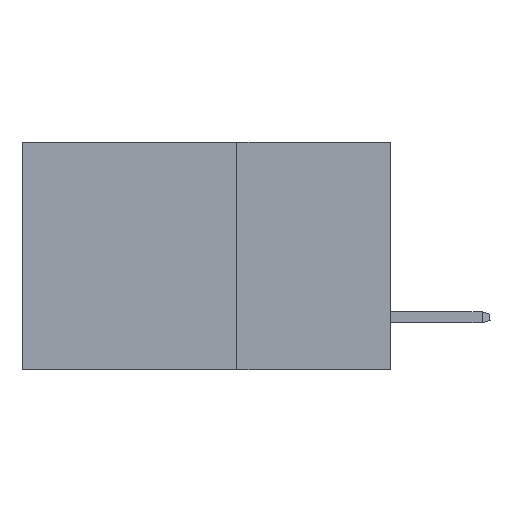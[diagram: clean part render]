
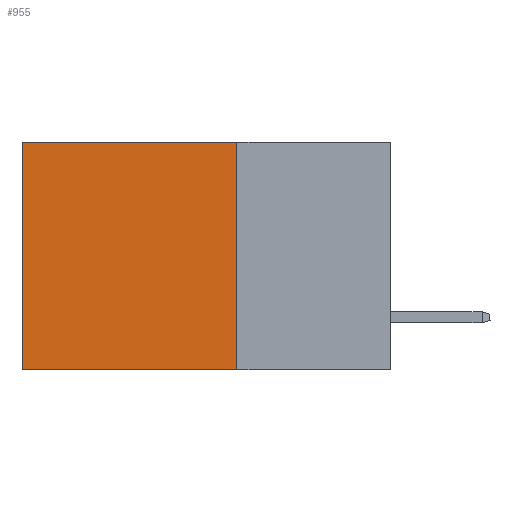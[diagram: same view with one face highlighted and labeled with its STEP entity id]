
A CAD part, left-side view. The second image highlights one B-rep face of the part: STEP entity #955.
In plain terms, the highlighted planar face has unit normal (-1, 0, 0).
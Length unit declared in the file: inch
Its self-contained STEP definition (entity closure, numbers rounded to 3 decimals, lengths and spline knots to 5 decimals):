
#955 = ADVANCED_FACE ( 'NONE', ( #3039 ), #11485, .F. ) ;
#1014 = EDGE_CURVE ( 'NONE', #9061, #15451, #6575, .T. ) ;
#3039 = FACE_OUTER_BOUND ( 'NONE', #24525, .T. ) ;
#3268 = VECTOR ( 'NONE', #10433, 39.37008 ) ;
#3573 = ORIENTED_EDGE ( 'NONE', *, *, #5496, .F. ) ;
#3801 = EDGE_CURVE ( 'NONE', #9061, #21072, #8751, .T. ) ;
#5016 = DIRECTION ( 'NONE',  ( 1., 0., 0. ) ) ;
#5496 = EDGE_CURVE ( 'NONE', #15451, #16793, #8081, .T. ) ;
#6575 = LINE ( 'NONE', #15434, #11398 ) ;
#7103 = VECTOR ( 'NONE', #8086, 39.37008 ) ;
#8081 = LINE ( 'NONE', #8127, #13527 ) ;
#8086 = DIRECTION ( 'NONE',  ( 0., 0., -1. ) ) ;
#8127 = CARTESIAN_POINT ( 'NONE',  ( 0.2875, 0.25, -0.37 ) ) ;
#8228 = ORIENTED_EDGE ( 'NONE', *, *, #3801, .T. ) ;
#8751 = LINE ( 'NONE', #21128, #3268 ) ;
#9061 = VERTEX_POINT ( 'NONE', #17352 ) ;
#10433 = DIRECTION ( 'NONE',  ( 0., 1., 0. ) ) ;
#10765 = ORIENTED_EDGE ( 'NONE', *, *, #24209, .T. ) ;
#11398 = VECTOR ( 'NONE', #17552, 39.37008 ) ;
#11485 = PLANE ( 'NONE',  #15212 ) ;
#13195 = CARTESIAN_POINT ( 'NONE',  ( 0.2875, 0.25, 0. ) ) ;
#13527 = VECTOR ( 'NONE', #26217, 39.37008 ) ;
#13822 = ORIENTED_EDGE ( 'NONE', *, *, #1014, .F. ) ;
#15212 = AXIS2_PLACEMENT_3D ( 'NONE', #13195, #5016, #25808 ) ;
#15434 = CARTESIAN_POINT ( 'NONE',  ( 0.2875, 0.25, 0. ) ) ;
#15451 = VERTEX_POINT ( 'NONE', #18130 ) ;
#16203 = CARTESIAN_POINT ( 'NONE',  ( 0.2875, 0.6, 0. ) ) ;
#16793 = VERTEX_POINT ( 'NONE', #17631 ) ;
#17352 = CARTESIAN_POINT ( 'NONE',  ( 0.2875, 0.25, 0. ) ) ;
#17552 = DIRECTION ( 'NONE',  ( 0., 0., -1. ) ) ;
#17631 = CARTESIAN_POINT ( 'NONE',  ( 0.2875, 0.6, -0.37 ) ) ;
#18130 = CARTESIAN_POINT ( 'NONE',  ( 0.2875, 0.25, -0.37 ) ) ;
#21072 = VERTEX_POINT ( 'NONE', #22028 ) ;
#21128 = CARTESIAN_POINT ( 'NONE',  ( 0.2875, 0.25, 0. ) ) ;
#22028 = CARTESIAN_POINT ( 'NONE',  ( 0.2875, 0.6, 0. ) ) ;
#24209 = EDGE_CURVE ( 'NONE', #21072, #16793, #25167, .T. ) ;
#24525 = EDGE_LOOP ( 'NONE', ( #10765, #3573, #13822, #8228 ) ) ;
#25167 = LINE ( 'NONE', #16203, #7103 ) ;
#25808 = DIRECTION ( 'NONE',  ( 0., 0., -1. ) ) ;
#26217 = DIRECTION ( 'NONE',  ( 0., 1., 0. ) ) ;
